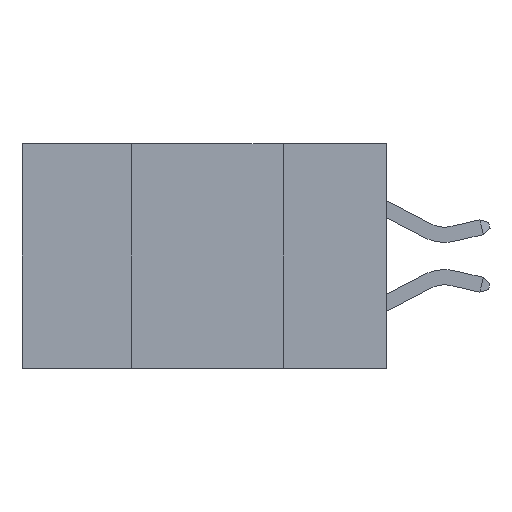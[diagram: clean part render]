
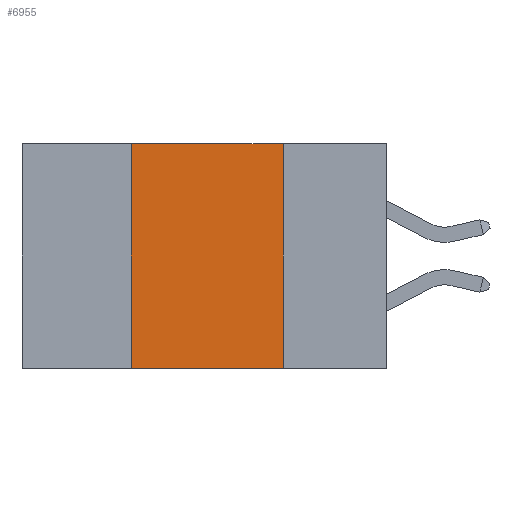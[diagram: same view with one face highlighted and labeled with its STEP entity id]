
A CAD part, left-side view. The second image highlights one B-rep face of the part: STEP entity #6955.
In plain terms, the highlighted planar face has unit normal (-1, 0, 0).
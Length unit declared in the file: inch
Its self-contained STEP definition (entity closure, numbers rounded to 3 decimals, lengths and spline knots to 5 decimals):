
#8 = FACE_OUTER_BOUND ( 'NONE', #8757, .T. ) ;
#901 = EDGE_CURVE ( 'NONE', #21024, #16419, #21428, .T. ) ;
#1239 = EDGE_CURVE ( 'NONE', #16419, #17645, #13915, .T. ) ;
#2040 = CARTESIAN_POINT ( 'NONE',  ( 0., 0.17, 0. ) ) ;
#2111 = DIRECTION ( 'NONE',  ( 0., -1., 0. ) ) ;
#4823 = EDGE_CURVE ( 'NONE', #8779, #21024, #19133, .T. ) ;
#5836 = DIRECTION ( 'NONE',  ( 0., -1., 0. ) ) ;
#6839 = ORIENTED_EDGE ( 'NONE', *, *, #31222, .T. ) ;
#6955 = ADVANCED_FACE ( 'NONE', ( #8 ), #12144, .F. ) ;
#8757 = EDGE_LOOP ( 'NONE', ( #12003, #25340, #16267, #6839 ) ) ;
#8779 = VERTEX_POINT ( 'NONE', #13441 ) ;
#9218 = VECTOR ( 'NONE', #5836, 39.37008 ) ;
#9339 = CARTESIAN_POINT ( 'NONE',  ( 0., 0.17, 0. ) ) ;
#10369 = CARTESIAN_POINT ( 'NONE',  ( 0., 0.6, 0. ) ) ;
#12003 = ORIENTED_EDGE ( 'NONE', *, *, #1239, .F. ) ;
#12144 = PLANE ( 'NONE',  #21558 ) ;
#12896 = CARTESIAN_POINT ( 'NONE',  ( 0., 0.17, -0.37 ) ) ;
#13441 = CARTESIAN_POINT ( 'NONE',  ( 0., 0.42, -0.37 ) ) ;
#13635 = DIRECTION ( 'NONE',  ( 0., 0., -1. ) ) ;
#13915 = LINE ( 'NONE', #2040, #19040 ) ;
#14624 = DIRECTION ( 'NONE',  ( 0., 0., -1. ) ) ;
#15956 = VECTOR ( 'NONE', #29492, 39.37008 ) ;
#15985 = CARTESIAN_POINT ( 'NONE',  ( 0., 0.6, -0.37 ) ) ;
#16267 = ORIENTED_EDGE ( 'NONE', *, *, #4823, .F. ) ;
#16419 = VERTEX_POINT ( 'NONE', #9339 ) ;
#17645 = VERTEX_POINT ( 'NONE', #12896 ) ;
#19040 = VECTOR ( 'NONE', #14624, 39.37008 ) ;
#19133 = LINE ( 'NONE', #19400, #15956 ) ;
#19400 = CARTESIAN_POINT ( 'NONE',  ( 0., 0.42, 0. ) ) ;
#21024 = VERTEX_POINT ( 'NONE', #22554 ) ;
#21428 = LINE ( 'NONE', #22269, #29746 ) ;
#21558 = AXIS2_PLACEMENT_3D ( 'NONE', #10369, #30521, #13635 ) ;
#22269 = CARTESIAN_POINT ( 'NONE',  ( 0., 0.6, 0. ) ) ;
#22554 = CARTESIAN_POINT ( 'NONE',  ( 0., 0.42, 0. ) ) ;
#25340 = ORIENTED_EDGE ( 'NONE', *, *, #901, .F. ) ;
#27474 = LINE ( 'NONE', #15985, #9218 ) ;
#29492 = DIRECTION ( 'NONE',  ( 0., 0., 1. ) ) ;
#29746 = VECTOR ( 'NONE', #2111, 39.37008 ) ;
#30521 = DIRECTION ( 'NONE',  ( 1., 0., 0. ) ) ;
#31222 = EDGE_CURVE ( 'NONE', #8779, #17645, #27474, .T. ) ;
